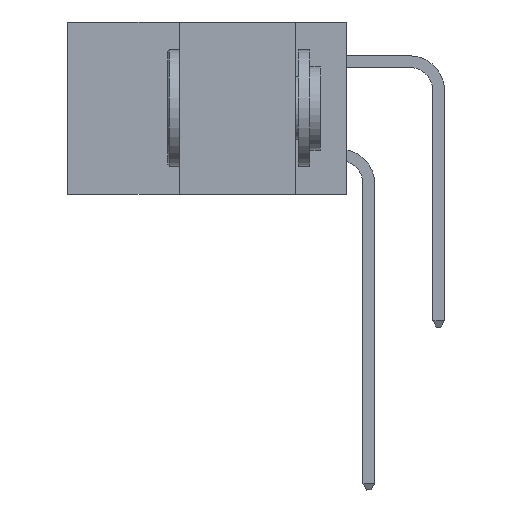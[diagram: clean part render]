
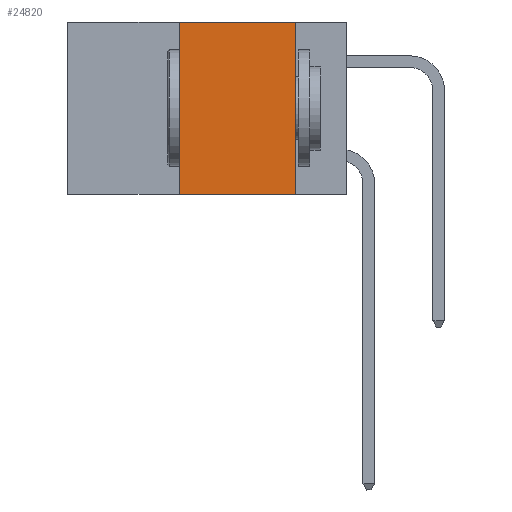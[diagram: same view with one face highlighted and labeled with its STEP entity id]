
A CAD part, left-side view. The second image highlights one B-rep face of the part: STEP entity #24820.
In plain terms, the highlighted planar face has unit normal (-1, 0, 0).
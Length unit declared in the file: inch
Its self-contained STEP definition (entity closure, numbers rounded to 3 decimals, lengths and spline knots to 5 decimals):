
#733 = EDGE_LOOP ( 'NONE', ( #23731, #13991, #16782, #2033 ) ) ;
#1115 = LINE ( 'NONE', #25885, #24217 ) ;
#2033 = ORIENTED_EDGE ( 'NONE', *, *, #26733, .T. ) ;
#2057 = CARTESIAN_POINT ( 'NONE',  ( 0., 0.6, 0. ) ) ;
#2239 = EDGE_CURVE ( 'NONE', #21018, #27990, #17995, .T. ) ;
#5275 = EDGE_CURVE ( 'NONE', #27990, #10470, #22603, .T. ) ;
#6929 = EDGE_CURVE ( 'NONE', #10470, #15113, #28374, .T. ) ;
#10470 = VERTEX_POINT ( 'NONE', #13031 ) ;
#10827 = VECTOR ( 'NONE', #19323, 39.37008 ) ;
#10875 = CARTESIAN_POINT ( 'NONE',  ( 0., 0.36, 0. ) ) ;
#12239 = CARTESIAN_POINT ( 'NONE',  ( 0., 0.6, 0. ) ) ;
#12445 = PLANE ( 'NONE',  #23795 ) ;
#12721 = DIRECTION ( 'NONE',  ( 0., -1., 0. ) ) ;
#12771 = CARTESIAN_POINT ( 'NONE',  ( 0., 0.11, 0. ) ) ;
#13031 = CARTESIAN_POINT ( 'NONE',  ( 0., 0.11, 0. ) ) ;
#13991 = ORIENTED_EDGE ( 'NONE', *, *, #5275, .F. ) ;
#14676 = DIRECTION ( 'NONE',  ( 0., 0., -1. ) ) ;
#15113 = VERTEX_POINT ( 'NONE', #15606 ) ;
#15606 = CARTESIAN_POINT ( 'NONE',  ( 0., 0.11, -0.37 ) ) ;
#16782 = ORIENTED_EDGE ( 'NONE', *, *, #2239, .F. ) ;
#16800 = VECTOR ( 'NONE', #24432, 39.37008 ) ;
#17995 = LINE ( 'NONE', #28661, #28250 ) ;
#19323 = DIRECTION ( 'NONE',  ( 0., 0., -1. ) ) ;
#19595 = FACE_OUTER_BOUND ( 'NONE', #733, .T. ) ;
#21018 = VERTEX_POINT ( 'NONE', #27225 ) ;
#22603 = LINE ( 'NONE', #2057, #16800 ) ;
#23731 = ORIENTED_EDGE ( 'NONE', *, *, #6929, .F. ) ;
#23795 = AXIS2_PLACEMENT_3D ( 'NONE', #12239, #27781, #14676 ) ;
#24217 = VECTOR ( 'NONE', #12721, 39.37008 ) ;
#24432 = DIRECTION ( 'NONE',  ( 0., -1., 0. ) ) ;
#24820 = ADVANCED_FACE ( 'NONE', ( #19595 ), #12445, .F. ) ;
#25885 = CARTESIAN_POINT ( 'NONE',  ( 0., 0.6, -0.37 ) ) ;
#26733 = EDGE_CURVE ( 'NONE', #21018, #15113, #1115, .T. ) ;
#27225 = CARTESIAN_POINT ( 'NONE',  ( 0., 0.36, -0.37 ) ) ;
#27781 = DIRECTION ( 'NONE',  ( 1., 0., 0. ) ) ;
#27990 = VERTEX_POINT ( 'NONE', #10875 ) ;
#28250 = VECTOR ( 'NONE', #28420, 39.37008 ) ;
#28374 = LINE ( 'NONE', #12771, #10827 ) ;
#28420 = DIRECTION ( 'NONE',  ( 0., 0., 1. ) ) ;
#28661 = CARTESIAN_POINT ( 'NONE',  ( 0., 0.36, 0. ) ) ;
